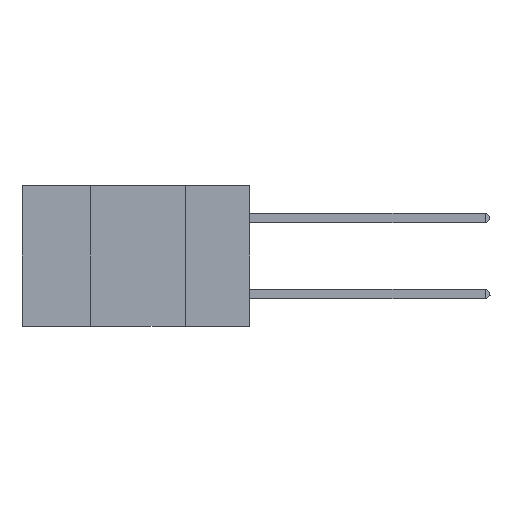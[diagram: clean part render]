
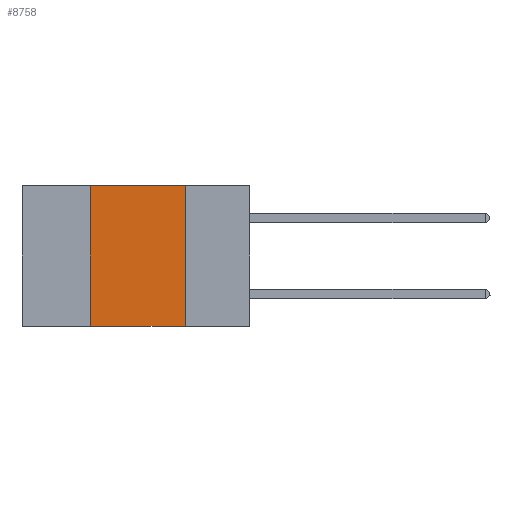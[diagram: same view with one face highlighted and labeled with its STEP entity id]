
A CAD part, left-side view. The second image highlights one B-rep face of the part: STEP entity #8758.
In plain terms, the highlighted planar face has unit normal (-1, 0, 0).
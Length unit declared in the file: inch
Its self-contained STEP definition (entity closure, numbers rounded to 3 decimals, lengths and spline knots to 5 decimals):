
#293 = CARTESIAN_POINT ( 'NONE',  ( 0., 0.6, 0. ) ) ;
#342 = DIRECTION ( 'NONE',  ( 0., 0., -1. ) ) ;
#541 = EDGE_CURVE ( 'NONE', #13199, #13078, #7840, .T. ) ;
#563 = EDGE_CURVE ( 'NONE', #6911, #9193, #3004, .T. ) ;
#775 = DIRECTION ( 'NONE',  ( 0., 0., -1. ) ) ;
#1248 = VECTOR ( 'NONE', #4793, 39.37008 ) ;
#1362 = DIRECTION ( 'NONE',  ( 0., -1., 0. ) ) ;
#1401 = CARTESIAN_POINT ( 'NONE',  ( 0., 0.17, -0.37 ) ) ;
#1483 = VECTOR ( 'NONE', #1362, 39.37008 ) ;
#1587 = EDGE_CURVE ( 'NONE', #13078, #6911, #16073, .T. ) ;
#1909 = LINE ( 'NONE', #11978, #9245 ) ;
#3004 = LINE ( 'NONE', #13618, #12875 ) ;
#3438 = ORIENTED_EDGE ( 'NONE', *, *, #563, .F. ) ;
#3458 = ORIENTED_EDGE ( 'NONE', *, *, #6460, .T. ) ;
#4643 = DIRECTION ( 'NONE',  ( 0., -1., 0. ) ) ;
#4793 = DIRECTION ( 'NONE',  ( 0., 0., 1. ) ) ;
#5178 = CARTESIAN_POINT ( 'NONE',  ( 0., 0.42, 0. ) ) ;
#5755 = AXIS2_PLACEMENT_3D ( 'NONE', #293, #13971, #342 ) ;
#6460 = EDGE_CURVE ( 'NONE', #13199, #9193, #1909, .T. ) ;
#6911 = VERTEX_POINT ( 'NONE', #7908 ) ;
#7840 = LINE ( 'NONE', #5178, #1248 ) ;
#7908 = CARTESIAN_POINT ( 'NONE',  ( 0., 0.17, 0. ) ) ;
#8758 = ADVANCED_FACE ( 'NONE', ( #13061 ), #15185, .F. ) ;
#9193 = VERTEX_POINT ( 'NONE', #1401 ) ;
#9245 = VECTOR ( 'NONE', #4643, 39.37008 ) ;
#9917 = EDGE_LOOP ( 'NONE', ( #3438, #12688, #10570, #3458 ) ) ;
#9964 = CARTESIAN_POINT ( 'NONE',  ( 0., 0.6, 0. ) ) ;
#10570 = ORIENTED_EDGE ( 'NONE', *, *, #541, .F. ) ;
#11978 = CARTESIAN_POINT ( 'NONE',  ( 0., 0.6, -0.37 ) ) ;
#12688 = ORIENTED_EDGE ( 'NONE', *, *, #1587, .F. ) ;
#12875 = VECTOR ( 'NONE', #775, 39.37008 ) ;
#13061 = FACE_OUTER_BOUND ( 'NONE', #9917, .T. ) ;
#13078 = VERTEX_POINT ( 'NONE', #14367 ) ;
#13199 = VERTEX_POINT ( 'NONE', #14815 ) ;
#13618 = CARTESIAN_POINT ( 'NONE',  ( 0., 0.17, 0. ) ) ;
#13971 = DIRECTION ( 'NONE',  ( 1., 0., 0. ) ) ;
#14367 = CARTESIAN_POINT ( 'NONE',  ( 0., 0.42, 0. ) ) ;
#14815 = CARTESIAN_POINT ( 'NONE',  ( 0., 0.42, -0.37 ) ) ;
#15185 = PLANE ( 'NONE',  #5755 ) ;
#16073 = LINE ( 'NONE', #9964, #1483 ) ;
